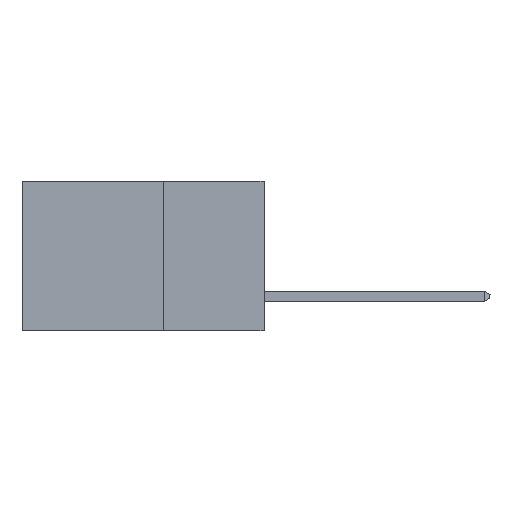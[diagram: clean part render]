
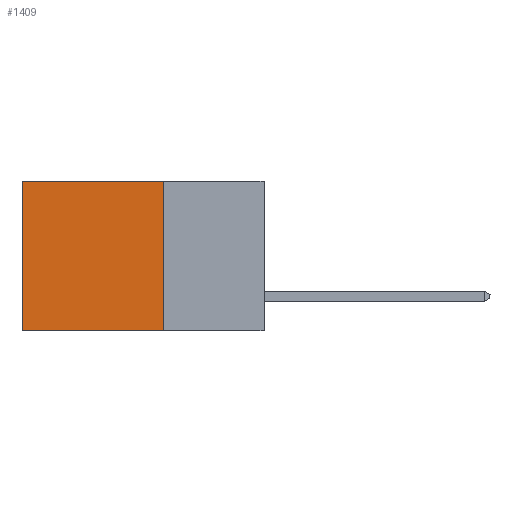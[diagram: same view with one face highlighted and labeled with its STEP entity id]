
A CAD part, left-side view. The second image highlights one B-rep face of the part: STEP entity #1409.
In plain terms, the highlighted planar face has unit normal (-1, 0, 0).
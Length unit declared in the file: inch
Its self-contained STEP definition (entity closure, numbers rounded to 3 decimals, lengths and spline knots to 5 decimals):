
#77 = VECTOR ( 'NONE', #23630, 39.37008 ) ;
#357 = ORIENTED_EDGE ( 'NONE', *, *, #7407, .T. ) ;
#1046 = FACE_OUTER_BOUND ( 'NONE', #22340, .T. ) ;
#1409 = ADVANCED_FACE ( 'NONE', ( #1046 ), #24994, .F. ) ;
#1609 = DIRECTION ( 'NONE',  ( 1., 0., 0. ) ) ;
#1763 = LINE ( 'NONE', #3702, #15728 ) ;
#2257 = CARTESIAN_POINT ( 'NONE',  ( 0.298, 0.6, 0. ) ) ;
#2414 = CARTESIAN_POINT ( 'NONE',  ( 0.298, 0.25, 0. ) ) ;
#3702 = CARTESIAN_POINT ( 'NONE',  ( 0.298, 0.25, -0.37 ) ) ;
#4915 = CARTESIAN_POINT ( 'NONE',  ( 0.298, 0.6, 0. ) ) ;
#5280 = LINE ( 'NONE', #2257, #77 ) ;
#5609 = ORIENTED_EDGE ( 'NONE', *, *, #9221, .F. ) ;
#6567 = VECTOR ( 'NONE', #14519, 39.37008 ) ;
#7407 = EDGE_CURVE ( 'NONE', #17033, #22978, #5280, .T. ) ;
#7843 = DIRECTION ( 'NONE',  ( 0., 1., 0. ) ) ;
#9221 = EDGE_CURVE ( 'NONE', #20630, #22978, #1763, .T. ) ;
#9527 = CARTESIAN_POINT ( 'NONE',  ( 0.298, 0.25, 0. ) ) ;
#12386 = VECTOR ( 'NONE', #19935, 39.37008 ) ;
#14519 = DIRECTION ( 'NONE',  ( 0., 0., -1. ) ) ;
#14987 = CARTESIAN_POINT ( 'NONE',  ( 0.298, 0.25, -0.37 ) ) ;
#15728 = VECTOR ( 'NONE', #7843, 39.37008 ) ;
#15934 = LINE ( 'NONE', #2414, #6567 ) ;
#17033 = VERTEX_POINT ( 'NONE', #4915 ) ;
#17973 = EDGE_CURVE ( 'NONE', #19538, #17033, #24523, .T. ) ;
#18006 = CARTESIAN_POINT ( 'NONE',  ( 0.298, 0.25, 0. ) ) ;
#19538 = VERTEX_POINT ( 'NONE', #21248 ) ;
#19636 = AXIS2_PLACEMENT_3D ( 'NONE', #9527, #1609, #22755 ) ;
#19935 = DIRECTION ( 'NONE',  ( 0., 1., 0. ) ) ;
#20469 = ORIENTED_EDGE ( 'NONE', *, *, #22046, .F. ) ;
#20630 = VERTEX_POINT ( 'NONE', #14987 ) ;
#21248 = CARTESIAN_POINT ( 'NONE',  ( 0.298, 0.25, 0. ) ) ;
#22046 = EDGE_CURVE ( 'NONE', #19538, #20630, #15934, .T. ) ;
#22340 = EDGE_LOOP ( 'NONE', ( #357, #5609, #20469, #23930 ) ) ;
#22755 = DIRECTION ( 'NONE',  ( 0., 0., -1. ) ) ;
#22978 = VERTEX_POINT ( 'NONE', #24613 ) ;
#23630 = DIRECTION ( 'NONE',  ( 0., 0., -1. ) ) ;
#23930 = ORIENTED_EDGE ( 'NONE', *, *, #17973, .T. ) ;
#24523 = LINE ( 'NONE', #18006, #12386 ) ;
#24613 = CARTESIAN_POINT ( 'NONE',  ( 0.298, 0.6, -0.37 ) ) ;
#24994 = PLANE ( 'NONE',  #19636 ) ;
